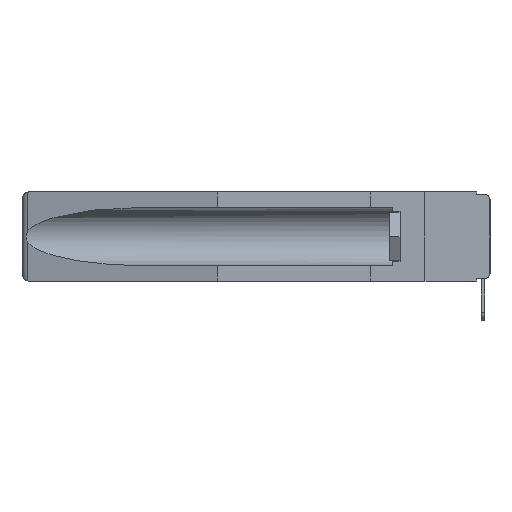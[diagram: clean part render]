
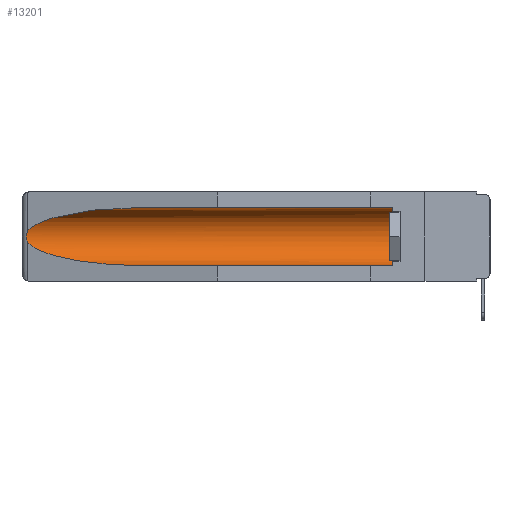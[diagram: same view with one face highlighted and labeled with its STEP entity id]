
A CAD part, left-side view. The second image highlights one B-rep face of the part: STEP entity #13201.
In plain terms, the highlighted cylindrical face has radius 2.857 mm (diameter 5.715 mm), a partial arc.
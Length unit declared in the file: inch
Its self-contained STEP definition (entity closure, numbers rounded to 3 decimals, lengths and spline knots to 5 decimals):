
#697 = CARTESIAN_POINT ( 'NONE',  ( 0.155, -0.30754, -0.059 ) ) ;
#729 =( BOUNDED_CURVE ( )  B_SPLINE_CURVE ( 3, ( #16098, #11053, #3103, #15943 ),
 .UNSPECIFIED., .F., .F. ) 
 B_SPLINE_CURVE_WITH_KNOTS ( ( 4, 4 ),
 ( 4.71239, 6.08839 ),
 .UNSPECIFIED. ) 
 CURVE ( )  GEOMETRIC_REPRESENTATION_ITEM ( )  RATIONAL_B_SPLINE_CURVE ( ( 1., 0.848, 0.848, 1. ) ) 
 REPRESENTATION_ITEM ( '' )  );
#1004 = CARTESIAN_POINT ( 'NONE',  ( 0.2675, 1.53308, -0.16763 ) ) ;
#1093 = LINE ( 'NONE', #17453, #16813 ) ;
#2384 = ORIENTED_EDGE ( 'NONE', *, *, #5096, .T. ) ;
#2470 = ORIENTED_EDGE ( 'NONE', *, *, #10060, .T. ) ;
#2848 = DIRECTION ( 'NONE',  ( 0., 1., 0. ) ) ;
#3103 = CARTESIAN_POINT ( 'NONE',  ( 0.25451, 1.48313, -0.09465 ) ) ;
#3219 = ORIENTED_EDGE ( 'NONE', *, *, #4876, .T. ) ;
#4327 = CARTESIAN_POINT ( 'NONE',  ( 0.26537, 1.52718, -0.19328 ) ) ;
#4876 = EDGE_CURVE ( 'NONE', #13812, #12416, #15182, .T. ) ;
#5096 = EDGE_CURVE ( 'NONE', #17088, #10018, #20215, .T. ) ;
#5415 =( BOUNDED_CURVE ( )  B_SPLINE_CURVE ( 3, ( #18432, #15185, #13538, #5461 ),
 .UNSPECIFIED., .F., .F. ) 
 B_SPLINE_CURVE_WITH_KNOTS ( ( 4, 4 ),
 ( 0.1948, 1.5708 ),
 .UNSPECIFIED. ) 
 CURVE ( )  GEOMETRIC_REPRESENTATION_ITEM ( )  RATIONAL_B_SPLINE_CURVE ( ( 1., 0.848, 0.848, 1. ) ) 
 REPRESENTATION_ITEM ( '' )  );
#5461 = CARTESIAN_POINT ( 'NONE',  ( 0.155, 1.07973, -0.284 ) ) ;
#5462 = DIRECTION ( 'NONE',  ( 0., -1., 0. ) ) ;
#5903 = CARTESIAN_POINT ( 'NONE',  ( 0.26655, 1.53094, -0.18657 ) ) ;
#6175 = CARTESIAN_POINT ( 'NONE',  ( 0.26537, 1.52718, -0.19328 ) ) ;
#9053 = VERTEX_POINT ( 'NONE', #18270 ) ;
#9064 = CARTESIAN_POINT ( 'NONE',  ( 0.26654, 1.53092, -0.15636 ) ) ;
#9948 = EDGE_CURVE ( 'NONE', #12416, #9053, #5415, .T. ) ;
#10018 = VERTEX_POINT ( 'NONE', #10335 ) ;
#10060 = EDGE_CURVE ( 'NONE', #10018, #15021, #11362, .T. ) ;
#10268 = DIRECTION ( 'NONE',  ( 0., 0., 1. ) ) ;
#10335 = CARTESIAN_POINT ( 'NONE',  ( 0.155, 0.126, -0.059 ) ) ;
#10705 = CARTESIAN_POINT ( 'NONE',  ( 0.2673, 1.5327, -0.16383 ) ) ;
#10966 = CARTESIAN_POINT ( 'NONE',  ( 0.26537, 1.52718, -0.14972 ) ) ;
#11053 = CARTESIAN_POINT ( 'NONE',  ( 0.21114, 1.30732, -0.059 ) ) ;
#11206 = CARTESIAN_POINT ( 'NONE',  ( 0.26537, 1.52718, -0.14972 ) ) ;
#11362 = LINE ( 'NONE', #697, #18718 ) ;
#11512 = AXIS2_PLACEMENT_3D ( 'NONE', #13513, #11871, #11804 ) ;
#11684 = FACE_OUTER_BOUND ( 'NONE', #11698, .T. ) ;
#11698 = EDGE_LOOP ( 'NONE', ( #14344, #3219, #13366, #12321, #2384, #2470 ) ) ;
#11804 = DIRECTION ( 'NONE',  ( 0., 0., 1. ) ) ;
#11871 = DIRECTION ( 'NONE',  ( 0., 1., 0. ) ) ;
#12321 = ORIENTED_EDGE ( 'NONE', *, *, #19033, .F. ) ;
#12339 = CARTESIAN_POINT ( 'NONE',  ( 0.2673, 1.53269, -0.17917 ) ) ;
#12416 = VERTEX_POINT ( 'NONE', #6175 ) ;
#13201 = ADVANCED_FACE ( 'NONE', ( #11684 ), #15752, .F. ) ;
#13267 = AXIS2_PLACEMENT_3D ( 'NONE', #15056, #5462, #10268 ) ;
#13366 = ORIENTED_EDGE ( 'NONE', *, *, #9948, .T. ) ;
#13513 = CARTESIAN_POINT ( 'NONE',  ( 0.155, -0.30754, -0.1715 ) ) ;
#13538 = CARTESIAN_POINT ( 'NONE',  ( 0.21114, 1.30732, -0.284 ) ) ;
#13812 = VERTEX_POINT ( 'NONE', #10966 ) ;
#14344 = ORIENTED_EDGE ( 'NONE', *, *, #17649, .T. ) ;
#15021 = VERTEX_POINT ( 'NONE', #19206 ) ;
#15056 = CARTESIAN_POINT ( 'NONE',  ( 0.155, 0.126, -0.1715 ) ) ;
#15182 = B_SPLINE_CURVE_WITH_KNOTS ( 'NONE', 3,
 ( #11206, #18728, #9064, #10705, #1004, #15607, #12339, #5903, #17233, #4327 ),
 .UNSPECIFIED., .F., .F.,
 ( 4, 2, 2, 2, 4 ),
 ( 0., 0.00029, 0.00058, 0.00087, 0.00117 ),
 .UNSPECIFIED. ) ;
#15185 = CARTESIAN_POINT ( 'NONE',  ( 0.25451, 1.48313, -0.24835 ) ) ;
#15607 = CARTESIAN_POINT ( 'NONE',  ( 0.2675, 1.53308, -0.17534 ) ) ;
#15752 = CYLINDRICAL_SURFACE ( 'NONE', #11512, 0.1125 ) ;
#15943 = CARTESIAN_POINT ( 'NONE',  ( 0.26537, 1.52718, -0.14972 ) ) ;
#16098 = CARTESIAN_POINT ( 'NONE',  ( 0.155, 1.07973, -0.059 ) ) ;
#16124 = CARTESIAN_POINT ( 'NONE',  ( 0.155, 0.126, -0.284 ) ) ;
#16813 = VECTOR ( 'NONE', #2848, 39.37008 ) ;
#17088 = VERTEX_POINT ( 'NONE', #16124 ) ;
#17233 = CARTESIAN_POINT ( 'NONE',  ( 0.26597, 1.5296, -0.19026 ) ) ;
#17453 = CARTESIAN_POINT ( 'NONE',  ( 0.155, -0.30754, -0.284 ) ) ;
#17649 = EDGE_CURVE ( 'NONE', #15021, #13812, #729, .T. ) ;
#18270 = CARTESIAN_POINT ( 'NONE',  ( 0.155, 1.07973, -0.284 ) ) ;
#18432 = CARTESIAN_POINT ( 'NONE',  ( 0.26537, 1.52718, -0.19328 ) ) ;
#18718 = VECTOR ( 'NONE', #18785, 39.37008 ) ;
#18728 = CARTESIAN_POINT ( 'NONE',  ( 0.26597, 1.52961, -0.15275 ) ) ;
#18785 = DIRECTION ( 'NONE',  ( 0., 1., 0. ) ) ;
#19033 = EDGE_CURVE ( 'NONE', #17088, #9053, #1093, .T. ) ;
#19206 = CARTESIAN_POINT ( 'NONE',  ( 0.155, 1.07973, -0.059 ) ) ;
#20215 = CIRCLE ( 'NONE', #13267, 0.1125 ) ;
